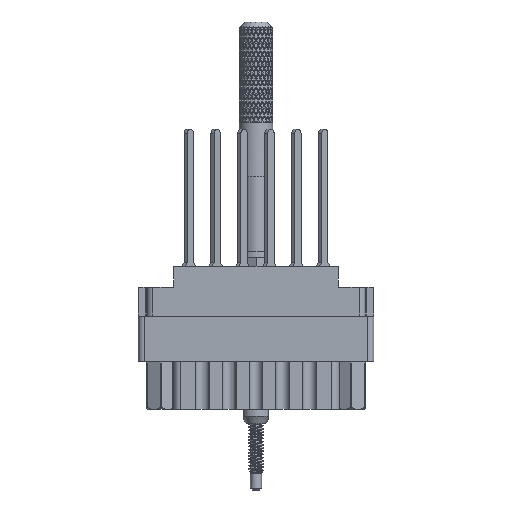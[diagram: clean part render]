
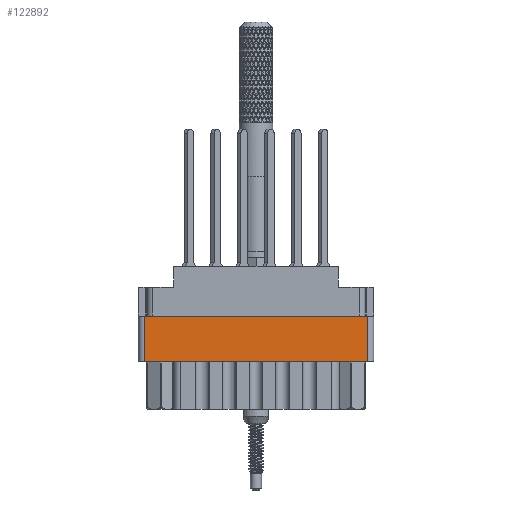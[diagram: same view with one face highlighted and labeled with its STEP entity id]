
A CAD part, front view. The second image highlights one B-rep face of the part: STEP entity #122892.
In plain terms, the highlighted planar face has unit normal (0, -1, 0).
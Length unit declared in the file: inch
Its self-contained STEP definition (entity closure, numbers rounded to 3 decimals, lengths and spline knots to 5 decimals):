
#2900 = CARTESIAN_POINT ( 'NONE',  ( 0.624, -0.343, -0.798 ) ) ;
#10610 = CARTESIAN_POINT ( 'NONE',  ( -0.624, -0.343, -0.277 ) ) ;
#24322 = CARTESIAN_POINT ( 'NONE',  ( -0.624, -0.343, -0.798 ) ) ;
#24471 = DIRECTION ( 'NONE',  ( -1., 0., 0. ) ) ;
#25285 = DIRECTION ( 'NONE',  ( 0., -1., 0. ) ) ;
#32344 = EDGE_LOOP ( 'NONE', ( #72089, #144043, #86405, #141159 ) ) ;
#39015 = CARTESIAN_POINT ( 'NONE',  ( 0.624, -0.343, -0.529 ) ) ;
#39668 = EDGE_CURVE ( 'NONE', #151130, #129585, #47540, .T. ) ;
#40803 = FACE_OUTER_BOUND ( 'NONE', #32344, .T. ) ;
#45502 = CARTESIAN_POINT ( 'NONE',  ( -0.656, -0.343, -0.277 ) ) ;
#47540 = LINE ( 'NONE', #2900, #151767 ) ;
#52074 = EDGE_CURVE ( 'NONE', #160428, #129585, #148459, .T. ) ;
#56266 = CARTESIAN_POINT ( 'NONE',  ( 0.624, -0.343, -0.529 ) ) ;
#62105 = DIRECTION ( 'NONE',  ( 0., 0., 1. ) ) ;
#72089 = ORIENTED_EDGE ( 'NONE', *, *, #183864, .F. ) ;
#86405 = ORIENTED_EDGE ( 'NONE', *, *, #39668, .T. ) ;
#94907 = VECTOR ( 'NONE', #170112, 39.37008 ) ;
#95391 = LINE ( 'NONE', #154619, #94907 ) ;
#98417 = CARTESIAN_POINT ( 'NONE',  ( 0.624, -0.343, -0.277 ) ) ;
#100009 = DIRECTION ( 'NONE',  ( 0., 0., -1. ) ) ;
#106064 = EDGE_CURVE ( 'NONE', #151130, #130434, #112815, .T. ) ;
#112815 = LINE ( 'NONE', #39015, #130725 ) ;
#122892 = ADVANCED_FACE ( 'NONE', ( #40803 ), #190309, .T. ) ;
#129585 = VERTEX_POINT ( 'NONE', #98417 ) ;
#130434 = VERTEX_POINT ( 'NONE', #143544 ) ;
#130725 = VECTOR ( 'NONE', #24471, 39.37008 ) ;
#140578 = DIRECTION ( 'NONE',  ( 1., 0., 0. ) ) ;
#141159 = ORIENTED_EDGE ( 'NONE', *, *, #52074, .F. ) ;
#143544 = CARTESIAN_POINT ( 'NONE',  ( -0.624, -0.343, -0.529 ) ) ;
#144043 = ORIENTED_EDGE ( 'NONE', *, *, #106064, .F. ) ;
#148459 = LINE ( 'NONE', #45502, #163976 ) ;
#151130 = VERTEX_POINT ( 'NONE', #56266 ) ;
#151767 = VECTOR ( 'NONE', #62105, 39.37008 ) ;
#154619 = CARTESIAN_POINT ( 'NONE',  ( -0.624, -0.343, -0.798 ) ) ;
#160428 = VERTEX_POINT ( 'NONE', #10610 ) ;
#161197 = AXIS2_PLACEMENT_3D ( 'NONE', #24322, #25285, #100009 ) ;
#163976 = VECTOR ( 'NONE', #140578, 39.37008 ) ;
#170112 = DIRECTION ( 'NONE',  ( 0., 0., 1. ) ) ;
#183864 = EDGE_CURVE ( 'NONE', #130434, #160428, #95391, .T. ) ;
#190309 = PLANE ( 'NONE',  #161197 ) ;
